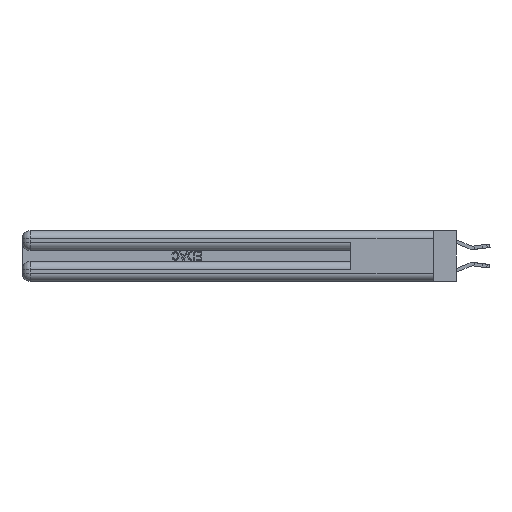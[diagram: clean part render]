
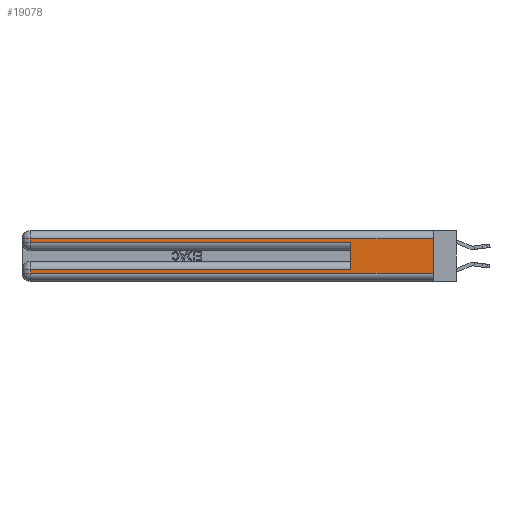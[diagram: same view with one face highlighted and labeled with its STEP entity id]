
A CAD part, left-side view. The second image highlights one B-rep face of the part: STEP entity #19078.
In plain terms, the highlighted planar face has unit normal (-1, 0, 0).
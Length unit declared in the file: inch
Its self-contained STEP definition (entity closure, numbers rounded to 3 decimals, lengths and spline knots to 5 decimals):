
#75 = VERTEX_POINT ( 'NONE', #5498 ) ;
#647 = CARTESIAN_POINT ( 'NONE',  ( 0., 2.94, 0.37 ) ) ;
#1418 = CARTESIAN_POINT ( 'NONE',  ( 0., 0., 0.085 ) ) ;
#1430 = VECTOR ( 'NONE', #27425, 39.37008 ) ;
#4547 = EDGE_CURVE ( 'NONE', #27714, #6107, #27464, .T. ) ;
#5498 = CARTESIAN_POINT ( 'NONE',  ( 0., 0., 0.06 ) ) ;
#5600 = ORIENTED_EDGE ( 'NONE', *, *, #7579, .T. ) ;
#5782 = EDGE_CURVE ( 'NONE', #10453, #75, #19333, .T. ) ;
#5831 = VECTOR ( 'NONE', #9356, 39.37008 ) ;
#5944 = VECTOR ( 'NONE', #10045, 39.37008 ) ;
#6107 = VERTEX_POINT ( 'NONE', #20104 ) ;
#6612 = DIRECTION ( 'NONE',  ( 0., 0., -1. ) ) ;
#6712 = VECTOR ( 'NONE', #7901, 39.37008 ) ;
#6768 = CARTESIAN_POINT ( 'NONE',  ( 0., 2.94, 0.285 ) ) ;
#7022 = EDGE_CURVE ( 'NONE', #9888, #75, #17287, .T. ) ;
#7160 = CARTESIAN_POINT ( 'NONE',  ( 0., 0., 0.37 ) ) ;
#7579 = EDGE_CURVE ( 'NONE', #20356, #10453, #17263, .T. ) ;
#7901 = DIRECTION ( 'NONE',  ( 0., 1., 0. ) ) ;
#8004 = LINE ( 'NONE', #26397, #13730 ) ;
#8551 = AXIS2_PLACEMENT_3D ( 'NONE', #21553, #19484, #6612 ) ;
#8921 = ORIENTED_EDGE ( 'NONE', *, *, #9747, .T. ) ;
#9356 = DIRECTION ( 'NONE',  ( 0., 0., -1. ) ) ;
#9747 = EDGE_CURVE ( 'NONE', #16480, #20356, #12481, .T. ) ;
#9888 = VERTEX_POINT ( 'NONE', #10556 ) ;
#9901 = CARTESIAN_POINT ( 'NONE',  ( 0., 0., 0.285 ) ) ;
#10045 = DIRECTION ( 'NONE',  ( 0., 0., -1. ) ) ;
#10453 = VERTEX_POINT ( 'NONE', #25388 ) ;
#10556 = CARTESIAN_POINT ( 'NONE',  ( 0., 0., 0.31 ) ) ;
#10905 = VECTOR ( 'NONE', #13646, 39.37008 ) ;
#11973 = EDGE_CURVE ( 'NONE', #9888, #20360, #21383, .T. ) ;
#12481 = LINE ( 'NONE', #1418, #6712 ) ;
#13598 = DIRECTION ( 'NONE',  ( 0., 0., 1. ) ) ;
#13646 = DIRECTION ( 'NONE',  ( 0., 0., -1. ) ) ;
#13730 = VECTOR ( 'NONE', #13598, 39.37008 ) ;
#13814 = CARTESIAN_POINT ( 'NONE',  ( 0., 0., 0.31 ) ) ;
#15694 = VECTOR ( 'NONE', #22422, 39.37008 ) ;
#15713 = ORIENTED_EDGE ( 'NONE', *, *, #7022, .F. ) ;
#15880 = EDGE_LOOP ( 'NONE', ( #15713, #17264, #27463, #23847, #20608, #8921, #5600, #18416 ) ) ;
#16480 = VERTEX_POINT ( 'NONE', #25326 ) ;
#17263 = LINE ( 'NONE', #647, #10905 ) ;
#17264 = ORIENTED_EDGE ( 'NONE', *, *, #11973, .T. ) ;
#17287 = LINE ( 'NONE', #7160, #5831 ) ;
#17328 = PLANE ( 'NONE',  #8551 ) ;
#17739 = FACE_OUTER_BOUND ( 'NONE', #15880, .T. ) ;
#18416 = ORIENTED_EDGE ( 'NONE', *, *, #5782, .T. ) ;
#19078 = ADVANCED_FACE ( 'NONE', ( #17739 ), #17328, .F. ) ;
#19223 = EDGE_CURVE ( 'NONE', #16480, #6107, #8004, .T. ) ;
#19333 = LINE ( 'NONE', #23125, #1430 ) ;
#19340 = EDGE_CURVE ( 'NONE', #20360, #27714, #23752, .T. ) ;
#19484 = DIRECTION ( 'NONE',  ( 1., 0., 0. ) ) ;
#20104 = CARTESIAN_POINT ( 'NONE',  ( 0., 0.6, 0.285 ) ) ;
#20356 = VERTEX_POINT ( 'NONE', #21681 ) ;
#20360 = VERTEX_POINT ( 'NONE', #23812 ) ;
#20608 = ORIENTED_EDGE ( 'NONE', *, *, #19223, .F. ) ;
#21383 = LINE ( 'NONE', #13814, #15694 ) ;
#21553 = CARTESIAN_POINT ( 'NONE',  ( 0., 0., 0.37 ) ) ;
#21681 = CARTESIAN_POINT ( 'NONE',  ( 0., 2.94, 0.085 ) ) ;
#22422 = DIRECTION ( 'NONE',  ( 0., 1., 0. ) ) ;
#22868 = CARTESIAN_POINT ( 'NONE',  ( 0., 2.94, 0.37 ) ) ;
#23125 = CARTESIAN_POINT ( 'NONE',  ( 0., 0., 0.06 ) ) ;
#23752 = LINE ( 'NONE', #22868, #5944 ) ;
#23812 = CARTESIAN_POINT ( 'NONE',  ( 0., 2.94, 0.31 ) ) ;
#23847 = ORIENTED_EDGE ( 'NONE', *, *, #4547, .T. ) ;
#24860 = DIRECTION ( 'NONE',  ( 0., -1., 0. ) ) ;
#25326 = CARTESIAN_POINT ( 'NONE',  ( 0., 0.6, 0.085 ) ) ;
#25388 = CARTESIAN_POINT ( 'NONE',  ( 0., 2.94, 0.06 ) ) ;
#26397 = CARTESIAN_POINT ( 'NONE',  ( 0., 0.6, 0.145 ) ) ;
#26779 = VECTOR ( 'NONE', #24860, 39.37008 ) ;
#27425 = DIRECTION ( 'NONE',  ( 0., -1., 0. ) ) ;
#27463 = ORIENTED_EDGE ( 'NONE', *, *, #19340, .T. ) ;
#27464 = LINE ( 'NONE', #9901, #26779 ) ;
#27714 = VERTEX_POINT ( 'NONE', #6768 ) ;
